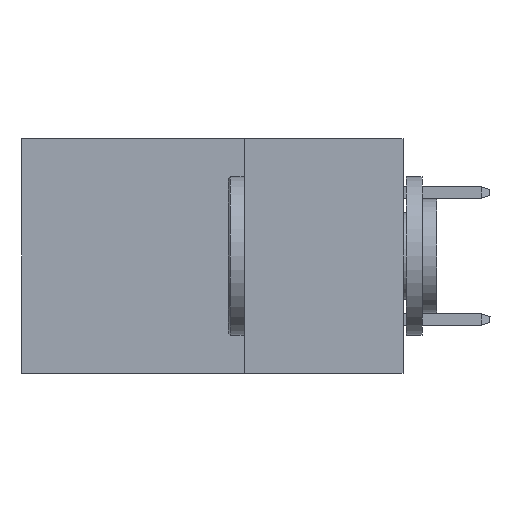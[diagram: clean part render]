
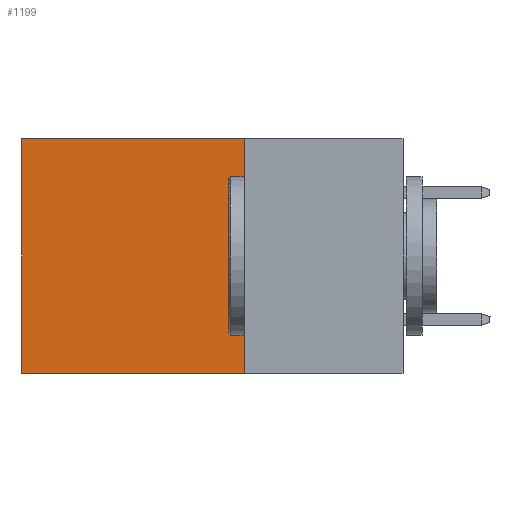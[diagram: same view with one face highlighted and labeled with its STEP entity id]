
A CAD part, left-side view. The second image highlights one B-rep face of the part: STEP entity #1199.
In plain terms, the highlighted planar face has unit normal (-1, 0, 0).
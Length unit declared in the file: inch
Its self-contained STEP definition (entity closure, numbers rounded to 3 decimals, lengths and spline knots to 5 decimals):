
#302 = EDGE_CURVE ( 'NONE', #14223, #15404, #9789, .T. ) ;
#1062 = CARTESIAN_POINT ( 'NONE',  ( 0.2875, 0.25, 0. ) ) ;
#1170 = VERTEX_POINT ( 'NONE', #14074 ) ;
#1199 = ADVANCED_FACE ( 'NONE', ( #13821 ), #3447, .F. ) ;
#1698 = EDGE_CURVE ( 'NONE', #10084, #15404, #11300, .T. ) ;
#2910 = CARTESIAN_POINT ( 'NONE',  ( 0.2875, 0.6, -0.37 ) ) ;
#3232 = VECTOR ( 'NONE', #6131, 39.37008 ) ;
#3447 = PLANE ( 'NONE',  #11694 ) ;
#4384 = CARTESIAN_POINT ( 'NONE',  ( 0.2875, 0.25, 0. ) ) ;
#4867 = ORIENTED_EDGE ( 'NONE', *, *, #1698, .T. ) ;
#5775 = ORIENTED_EDGE ( 'NONE', *, *, #6025, .T. ) ;
#6025 = EDGE_CURVE ( 'NONE', #1170, #10084, #16040, .T. ) ;
#6131 = DIRECTION ( 'NONE',  ( 0., 1., 0. ) ) ;
#7521 = EDGE_CURVE ( 'NONE', #1170, #14223, #13960, .T. ) ;
#7531 = DIRECTION ( 'NONE',  ( 1., 0., 0. ) ) ;
#8554 = DIRECTION ( 'NONE',  ( 0., 0., -1. ) ) ;
#8643 = CARTESIAN_POINT ( 'NONE',  ( 0.2875, 0.25, 0. ) ) ;
#8764 = DIRECTION ( 'NONE',  ( 0., 0., -1. ) ) ;
#9789 = LINE ( 'NONE', #14982, #3232 ) ;
#10084 = VERTEX_POINT ( 'NONE', #11536 ) ;
#10885 = ORIENTED_EDGE ( 'NONE', *, *, #302, .F. ) ;
#11300 = LINE ( 'NONE', #16516, #15486 ) ;
#11536 = CARTESIAN_POINT ( 'NONE',  ( 0.2875, 0.6, 0. ) ) ;
#11694 = AXIS2_PLACEMENT_3D ( 'NONE', #8643, #7531, #8554 ) ;
#12344 = DIRECTION ( 'NONE',  ( 0., 1., 0. ) ) ;
#13796 = DIRECTION ( 'NONE',  ( 0., 0., -1. ) ) ;
#13821 = FACE_OUTER_BOUND ( 'NONE', #15502, .T. ) ;
#13960 = LINE ( 'NONE', #1062, #15957 ) ;
#14074 = CARTESIAN_POINT ( 'NONE',  ( 0.2875, 0.25, 0. ) ) ;
#14223 = VERTEX_POINT ( 'NONE', #16409 ) ;
#14982 = CARTESIAN_POINT ( 'NONE',  ( 0.2875, 0.25, -0.37 ) ) ;
#15128 = VECTOR ( 'NONE', #12344, 39.37008 ) ;
#15404 = VERTEX_POINT ( 'NONE', #2910 ) ;
#15486 = VECTOR ( 'NONE', #8764, 39.37008 ) ;
#15502 = EDGE_LOOP ( 'NONE', ( #4867, #10885, #15771, #5775 ) ) ;
#15771 = ORIENTED_EDGE ( 'NONE', *, *, #7521, .F. ) ;
#15957 = VECTOR ( 'NONE', #13796, 39.37008 ) ;
#16040 = LINE ( 'NONE', #4384, #15128 ) ;
#16409 = CARTESIAN_POINT ( 'NONE',  ( 0.2875, 0.25, -0.37 ) ) ;
#16516 = CARTESIAN_POINT ( 'NONE',  ( 0.2875, 0.6, 0. ) ) ;
